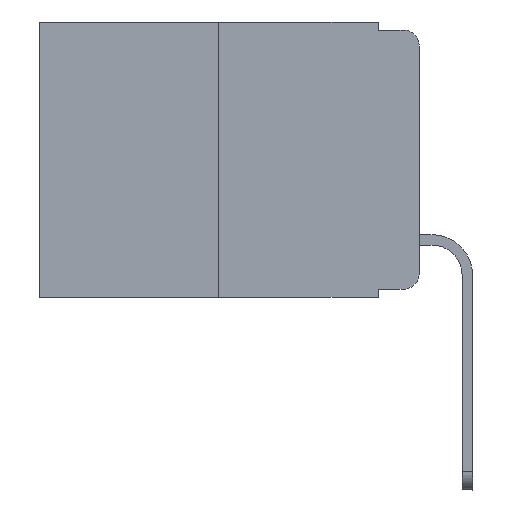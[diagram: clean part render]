
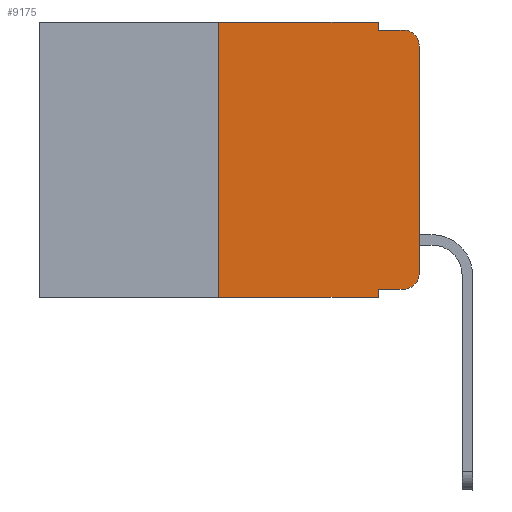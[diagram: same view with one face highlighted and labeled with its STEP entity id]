
A CAD part, left-side view. The second image highlights one B-rep face of the part: STEP entity #9175.
In plain terms, the highlighted planar face has unit normal (-1, 0, 0).
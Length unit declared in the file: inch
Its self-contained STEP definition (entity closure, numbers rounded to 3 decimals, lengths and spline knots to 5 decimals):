
#265 = CARTESIAN_POINT ( 'NONE',  ( 0., 0.051, 0. ) ) ;
#280 = VERTEX_POINT ( 'NONE', #11134 ) ;
#754 = DIRECTION ( 'NONE',  ( 0., 0., 1. ) ) ;
#835 = CARTESIAN_POINT ( 'NONE',  ( 0., 0.473, 0. ) ) ;
#965 = CARTESIAN_POINT ( 'NONE',  ( 0., 0.25, 0. ) ) ;
#1541 = LINE ( 'NONE', #14695, #1657 ) ;
#1550 = ORIENTED_EDGE ( 'NONE', *, *, #17135, .F. ) ;
#1657 = VECTOR ( 'NONE', #1859, 39.37008 ) ;
#1859 = DIRECTION ( 'NONE',  ( 0., -1., 0. ) ) ;
#2043 = CARTESIAN_POINT ( 'NONE',  ( 0., 0.051, -0.333 ) ) ;
#2464 = EDGE_CURVE ( 'NONE', #280, #2541, #7514, .T. ) ;
#2541 = VERTEX_POINT ( 'NONE', #4097 ) ;
#2786 = LINE ( 'NONE', #11350, #11395 ) ;
#2974 = EDGE_CURVE ( 'NONE', #4338, #7557, #15413, .T. ) ;
#3189 = CARTESIAN_POINT ( 'NONE',  ( 0., 0.25, 0. ) ) ;
#3358 = AXIS2_PLACEMENT_3D ( 'NONE', #3381, #9927, #4874 ) ;
#3381 = CARTESIAN_POINT ( 'NONE',  ( 0., 0.02, -0.03 ) ) ;
#3912 = DIRECTION ( 'NONE',  ( 0., 0., -1. ) ) ;
#4097 = CARTESIAN_POINT ( 'NONE',  ( 0., 0.02, -0.01 ) ) ;
#4270 = DIRECTION ( 'NONE',  ( -1., 0., 0. ) ) ;
#4338 = VERTEX_POINT ( 'NONE', #13060 ) ;
#4866 = LINE ( 'NONE', #265, #15126 ) ;
#4874 = DIRECTION ( 'NONE',  ( 0., 0., -1. ) ) ;
#4915 = ORIENTED_EDGE ( 'NONE', *, *, #9972, .T. ) ;
#5310 = LINE ( 'NONE', #9259, #9323 ) ;
#5322 = EDGE_CURVE ( 'NONE', #4338, #18151, #1541, .T. ) ;
#5359 = DIRECTION ( 'NONE',  ( 0., -1., 0. ) ) ;
#5512 = LINE ( 'NONE', #7231, #17507 ) ;
#6227 = VECTOR ( 'NONE', #5359, 39.37008 ) ;
#6574 = EDGE_CURVE ( 'NONE', #8567, #2541, #7819, .T. ) ;
#6757 = CARTESIAN_POINT ( 'NONE',  ( 0., 0.473, 0. ) ) ;
#6978 = LINE ( 'NONE', #6757, #6227 ) ;
#7157 = DIRECTION ( 'NONE',  ( 1., 0., 0. ) ) ;
#7231 = CARTESIAN_POINT ( 'NONE',  ( 0., 0.051, 0. ) ) ;
#7514 = LINE ( 'NONE', #12345, #15252 ) ;
#7557 = VERTEX_POINT ( 'NONE', #3189 ) ;
#7819 = CIRCLE ( 'NONE', #3358, 0.02 ) ;
#8393 = CARTESIAN_POINT ( 'NONE',  ( 0., 0.02, -0.333 ) ) ;
#8473 = CARTESIAN_POINT ( 'NONE',  ( 0., 0., -0.03 ) ) ;
#8567 = VERTEX_POINT ( 'NONE', #8473 ) ;
#8593 = VERTEX_POINT ( 'NONE', #18105 ) ;
#9175 = ADVANCED_FACE ( 'NONE', ( #15504 ), #13796, .F. ) ;
#9259 = CARTESIAN_POINT ( 'NONE',  ( 0., 0.051, -0.333 ) ) ;
#9323 = VECTOR ( 'NONE', #15770, 39.37008 ) ;
#9329 = DIRECTION ( 'NONE',  ( 0., 0., 1. ) ) ;
#9927 = DIRECTION ( 'NONE',  ( -1., 0., 0. ) ) ;
#9972 = EDGE_CURVE ( 'NONE', #17034, #16665, #5310, .T. ) ;
#10174 = DIRECTION ( 'NONE',  ( 0., 0., -1. ) ) ;
#11084 = CARTESIAN_POINT ( 'NONE',  ( 0., 0.051, -0.343 ) ) ;
#11134 = CARTESIAN_POINT ( 'NONE',  ( 0., 0.051, -0.01 ) ) ;
#11325 = CARTESIAN_POINT ( 'NONE',  ( 0., 0.051, 0. ) ) ;
#11350 = CARTESIAN_POINT ( 'NONE',  ( 0., 0., 0. ) ) ;
#11395 = VECTOR ( 'NONE', #9329, 39.37008 ) ;
#11424 = DIRECTION ( 'NONE',  ( 0., 0., -1. ) ) ;
#12034 = ORIENTED_EDGE ( 'NONE', *, *, #12172, .T. ) ;
#12172 = EDGE_CURVE ( 'NONE', #8593, #8567, #2786, .T. ) ;
#12345 = CARTESIAN_POINT ( 'NONE',  ( 0., 0.051, -0.01 ) ) ;
#12524 = VECTOR ( 'NONE', #754, 39.37008 ) ;
#12644 = DIRECTION ( 'NONE',  ( 0., 0., -1. ) ) ;
#12751 = CARTESIAN_POINT ( 'NONE',  ( 0., 0.02, -0.313 ) ) ;
#13060 = CARTESIAN_POINT ( 'NONE',  ( 0., 0.25, -0.343 ) ) ;
#13088 = ORIENTED_EDGE ( 'NONE', *, *, #19048, .T. ) ;
#13249 = ORIENTED_EDGE ( 'NONE', *, *, #2464, .F. ) ;
#13395 = ORIENTED_EDGE ( 'NONE', *, *, #21057, .F. ) ;
#13526 = EDGE_LOOP ( 'NONE', ( #12034, #19692, #13249, #13395, #1550, #19305, #16268, #20667, #4915, #13088 ) ) ;
#13796 = PLANE ( 'NONE',  #17020 ) ;
#14695 = CARTESIAN_POINT ( 'NONE',  ( 0., 0.473, -0.343 ) ) ;
#14763 = VERTEX_POINT ( 'NONE', #11325 ) ;
#15086 = AXIS2_PLACEMENT_3D ( 'NONE', #12751, #4270, #12644 ) ;
#15126 = VECTOR ( 'NONE', #11424, 39.37008 ) ;
#15252 = VECTOR ( 'NONE', #20679, 39.37008 ) ;
#15413 = LINE ( 'NONE', #965, #12524 ) ;
#15504 = FACE_OUTER_BOUND ( 'NONE', #13526, .T. ) ;
#15770 = DIRECTION ( 'NONE',  ( 0., -1., 0. ) ) ;
#16268 = ORIENTED_EDGE ( 'NONE', *, *, #5322, .T. ) ;
#16665 = VERTEX_POINT ( 'NONE', #8393 ) ;
#17020 = AXIS2_PLACEMENT_3D ( 'NONE', #835, #7157, #10174 ) ;
#17034 = VERTEX_POINT ( 'NONE', #2043 ) ;
#17135 = EDGE_CURVE ( 'NONE', #7557, #14763, #6978, .T. ) ;
#17142 = CIRCLE ( 'NONE', #15086, 0.02 ) ;
#17507 = VECTOR ( 'NONE', #3912, 39.37008 ) ;
#17916 = EDGE_CURVE ( 'NONE', #17034, #18151, #4866, .T. ) ;
#18105 = CARTESIAN_POINT ( 'NONE',  ( 0., 0., -0.313 ) ) ;
#18151 = VERTEX_POINT ( 'NONE', #11084 ) ;
#19048 = EDGE_CURVE ( 'NONE', #16665, #8593, #17142, .T. ) ;
#19305 = ORIENTED_EDGE ( 'NONE', *, *, #2974, .F. ) ;
#19692 = ORIENTED_EDGE ( 'NONE', *, *, #6574, .T. ) ;
#20667 = ORIENTED_EDGE ( 'NONE', *, *, #17916, .F. ) ;
#20679 = DIRECTION ( 'NONE',  ( 0., -1., 0. ) ) ;
#21057 = EDGE_CURVE ( 'NONE', #14763, #280, #5512, .T. ) ;
